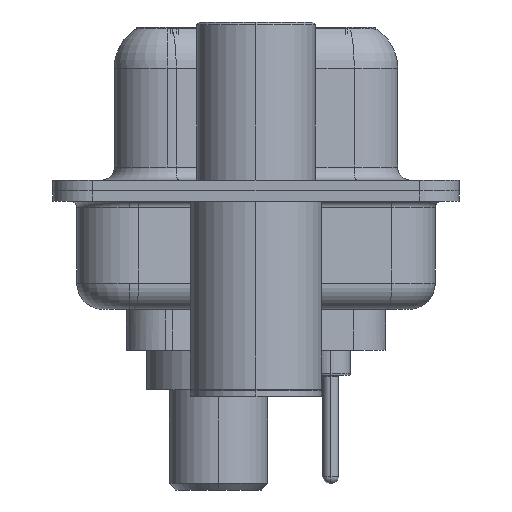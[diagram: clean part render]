
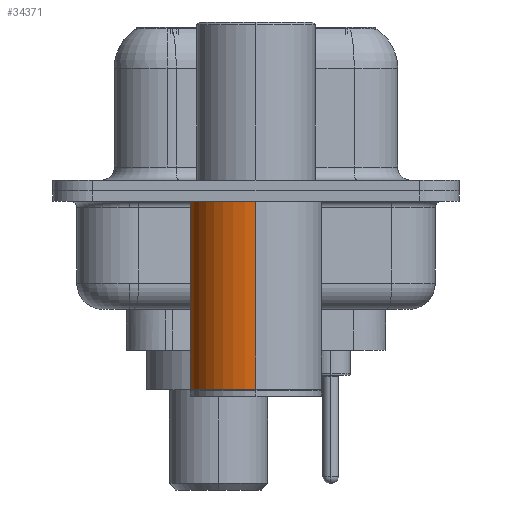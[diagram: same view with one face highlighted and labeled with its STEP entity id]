
A CAD part, left-side view. The second image highlights one B-rep face of the part: STEP entity #34371.
In plain terms, the highlighted cylindrical face has radius 2.5 mm (diameter 5 mm), a partial arc.
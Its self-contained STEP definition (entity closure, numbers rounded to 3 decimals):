
#478 = EDGE_LOOP ( 'NONE', ( #32692, #14830, #13832, #23139 ) ) ;
#2416 = CARTESIAN_POINT ( 'NONE',  ( 0., 0., 0.581 ) ) ;
#2665 = CARTESIAN_POINT ( 'NONE',  ( 0., 0., -0.4 ) ) ;
#3204 = EDGE_CURVE ( 'NONE', #27782, #15717, #19630, .T. ) ;
#5058 = CIRCLE ( 'NONE', #12042, 2.5 ) ;
#8049 = CARTESIAN_POINT ( 'NONE',  ( 2.5, 0., -7.525 ) ) ;
#9801 = EDGE_CURVE ( 'NONE', #17987, #21156, #26045, .T. ) ;
#10106 = AXIS2_PLACEMENT_3D ( 'NONE', #34077, #20770, #31499 ) ;
#12042 = AXIS2_PLACEMENT_3D ( 'NONE', #2665, #21659, #27106 ) ;
#13832 = ORIENTED_EDGE ( 'NONE', *, *, #34572, .F. ) ;
#14830 = ORIENTED_EDGE ( 'NONE', *, *, #3204, .T. ) ;
#15543 = CARTESIAN_POINT ( 'NONE',  ( 2.5, 0., -0.4 ) ) ;
#15717 = VERTEX_POINT ( 'NONE', #20544 ) ;
#15834 = EDGE_CURVE ( 'NONE', #17987, #27782, #21564, .T. ) ;
#17987 = VERTEX_POINT ( 'NONE', #8049 ) ;
#18629 = CARTESIAN_POINT ( 'NONE',  ( -2.5, 0., -7.525 ) ) ;
#19630 = LINE ( 'NONE', #21305, #25969 ) ;
#20544 = CARTESIAN_POINT ( 'NONE',  ( -2.5, 0., -0.4 ) ) ;
#20770 = DIRECTION ( 'NONE',  ( 0., 0., 1. ) ) ;
#20891 = AXIS2_PLACEMENT_3D ( 'NONE', #2416, #29244, #21309 ) ;
#21083 = FACE_OUTER_BOUND ( 'NONE', #478, .T. ) ;
#21156 = VERTEX_POINT ( 'NONE', #15543 ) ;
#21305 = CARTESIAN_POINT ( 'NONE',  ( -2.5, 0., 0.581 ) ) ;
#21309 = DIRECTION ( 'NONE',  ( 1., 0., 0. ) ) ;
#21564 = CIRCLE ( 'NONE', #10106, 2.5 ) ;
#21659 = DIRECTION ( 'NONE',  ( 0., 0., 1. ) ) ;
#23139 = ORIENTED_EDGE ( 'NONE', *, *, #9801, .F. ) ;
#23907 = DIRECTION ( 'NONE',  ( 0., 0., 1. ) ) ;
#25969 = VECTOR ( 'NONE', #23907, 1000. ) ;
#26045 = LINE ( 'NONE', #31207, #26896 ) ;
#26896 = VECTOR ( 'NONE', #31327, 1000. ) ;
#27106 = DIRECTION ( 'NONE',  ( 1., 0., 0. ) ) ;
#27782 = VERTEX_POINT ( 'NONE', #18629 ) ;
#29244 = DIRECTION ( 'NONE',  ( 0., 0., 1. ) ) ;
#31207 = CARTESIAN_POINT ( 'NONE',  ( 2.5, 0., 0.581 ) ) ;
#31327 = DIRECTION ( 'NONE',  ( 0., 0., 1. ) ) ;
#31499 = DIRECTION ( 'NONE',  ( 1., 0., 0. ) ) ;
#32692 = ORIENTED_EDGE ( 'NONE', *, *, #15834, .T. ) ;
#33270 = CYLINDRICAL_SURFACE ( 'NONE', #20891, 2.5 ) ;
#34077 = CARTESIAN_POINT ( 'NONE',  ( 0., 0., -7.525 ) ) ;
#34371 = ADVANCED_FACE ( 'NONE', ( #21083 ), #33270, .T. ) ;
#34572 = EDGE_CURVE ( 'NONE', #21156, #15717, #5058, .T. ) ;
